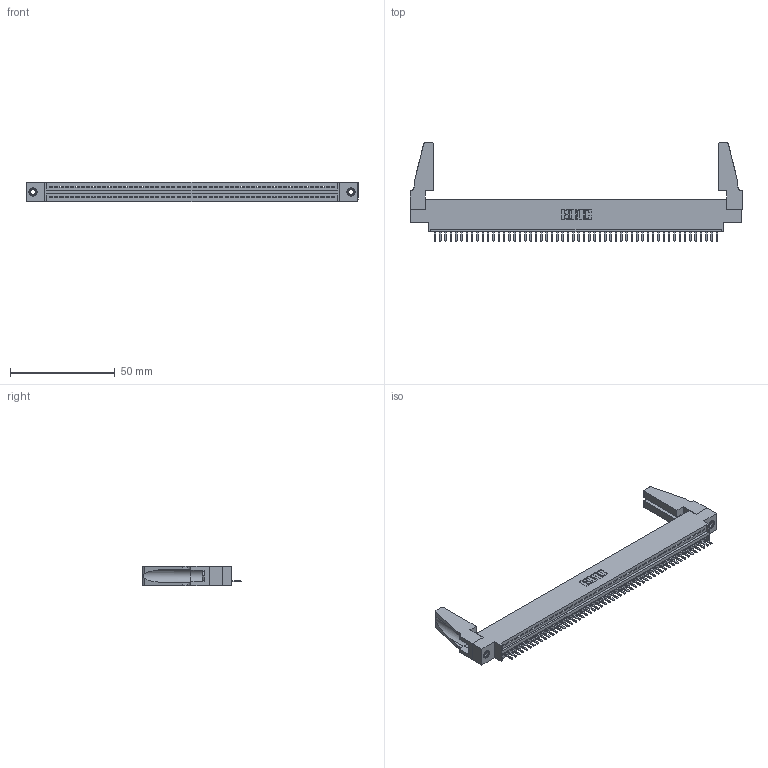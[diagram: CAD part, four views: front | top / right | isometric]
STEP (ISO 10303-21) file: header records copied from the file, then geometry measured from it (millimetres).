
FILE_DESCRIPTION (( 'STEP AP203' ), '1' );
FILE_NAME ('395-054-520-688.STEP', '2019-10-23T16:34:38', ( '' ), ( '' ), 'SwSTEP 2.0', 'SolidWorks 2016', '' );
FILE_SCHEMA (( 'CONFIG_CONTROL_DESIGN' ));
Length unit declared in the file: inch
Products named in the file (5): 345-292-001_345-293-120; 345-220-078_345-220-088; 345 Part_0.170 Offset - 0.156 Dia-TH; 395-054-520-688; 345-250-001_345-250-001-102
Assembly tree (59 placements, depth 2):
  395-054-520-688
    345 Part_0.170 Offset - 0.156 Dia-TH
    345-292-001_345-293-120  x54
    345-250-001_345-250-001-102  x2
    345-220-078_345-220-088  x2
Bounding box: 158.39 x 46.86 x 9.4 mm (x, y, z)
Volume: 18126.5 mm3; surface area: 22677 mm2
Topology: 59 solids, 59 shells, 3602 faces, 10603 edges, 6914 vertices
Faces by surface type: plane 2424, cylinder 1162, cone 12, torus 4
Entity records: 41420 total; most frequent: CARTESIAN_POINT 7176, ORIENTED_EDGE 7112, DIRECTION 6244, EDGE_CURVE 3556, LINE 3162, VECTOR 3162, VERTEX_POINT 2362, AXIS2_PLACEMENT_3D 1541
